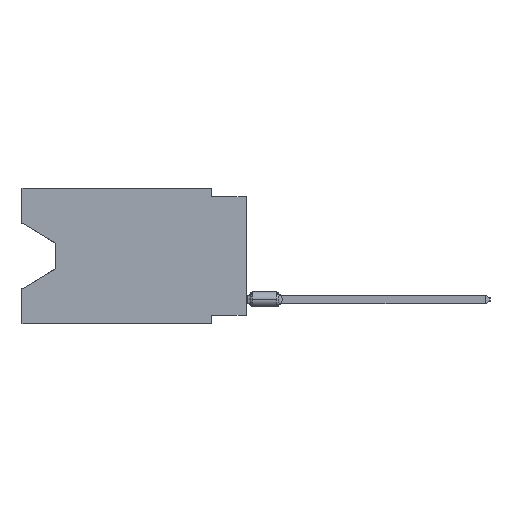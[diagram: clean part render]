
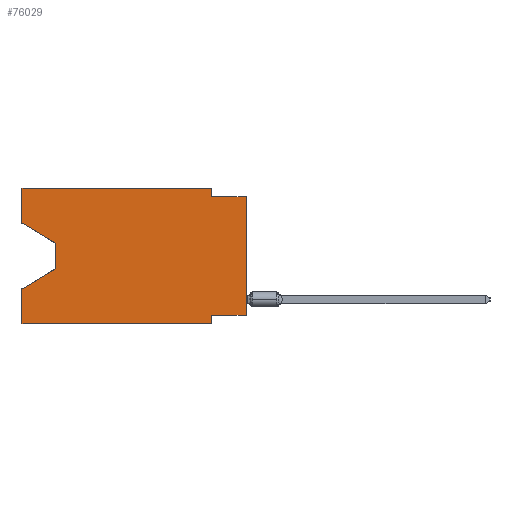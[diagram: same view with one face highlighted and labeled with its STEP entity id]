
A CAD part, left-side view. The second image highlights one B-rep face of the part: STEP entity #76029.
In plain terms, the highlighted planar face has unit normal (-1, 0, 0).
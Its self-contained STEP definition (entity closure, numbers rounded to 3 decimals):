
#23 = EDGE_CURVE ( 'NONE', #37314, #13199, #79784, .T. ) ;
#1327 = VECTOR ( 'NONE', #41392, 1000. ) ;
#2530 = VERTEX_POINT ( 'NONE', #23302 ) ;
#3319 = VERTEX_POINT ( 'NONE', #65923 ) ;
#4534 = VERTEX_POINT ( 'NONE', #23114 ) ;
#5900 = VECTOR ( 'NONE', #79385, 1000. ) ;
#6342 = LINE ( 'NONE', #75004, #16900 ) ;
#7025 = LINE ( 'NONE', #39284, #61425 ) ;
#7701 = EDGE_CURVE ( 'NONE', #2530, #56738, #6342, .T. ) ;
#9092 = LINE ( 'NONE', #40565, #30759 ) ;
#10693 = LINE ( 'NONE', #35314, #20684 ) ;
#11210 = CARTESIAN_POINT ( 'NONE',  ( 0., 16.383, 0. ) ) ;
#12800 = DIRECTION ( 'NONE',  ( 0., 0., 1. ) ) ;
#13199 = VERTEX_POINT ( 'NONE', #54015 ) ;
#13391 = VERTEX_POINT ( 'NONE', #25727 ) ;
#14161 = DIRECTION ( 'NONE',  ( 0., 0., -1. ) ) ;
#15362 = CARTESIAN_POINT ( 'NONE',  ( 0., 0., -0.635 ) ) ;
#16900 = VECTOR ( 'NONE', #24921, 1000. ) ;
#17189 = LINE ( 'NONE', #23638, #78007 ) ;
#18224 = PLANE ( 'NONE',  #79204 ) ;
#18334 = EDGE_CURVE ( 'NONE', #4534, #2530, #60759, .T. ) ;
#20684 = VECTOR ( 'NONE', #71680, 1000. ) ;
#20814 = DIRECTION ( 'NONE',  ( 0., 0.855, -0.519 ) ) ;
#21112 = VERTEX_POINT ( 'NONE', #76493 ) ;
#21815 = VERTEX_POINT ( 'NONE', #11210 ) ;
#22926 = ORIENTED_EDGE ( 'NONE', *, *, #48406, .T. ) ;
#23114 = CARTESIAN_POINT ( 'NONE',  ( 0., 0., -9.271 ) ) ;
#23302 = CARTESIAN_POINT ( 'NONE',  ( 0., 2.54, -9.271 ) ) ;
#23452 = EDGE_CURVE ( 'NONE', #35636, #56738, #17189, .T. ) ;
#23604 = CARTESIAN_POINT ( 'NONE',  ( 0., 16.383, 0. ) ) ;
#23638 = CARTESIAN_POINT ( 'NONE',  ( 0., 16.383, -9.906 ) ) ;
#24279 = CARTESIAN_POINT ( 'NONE',  ( 0., 16.383, -2.546 ) ) ;
#24784 = EDGE_CURVE ( 'NONE', #21815, #21112, #53457, .T. ) ;
#24921 = DIRECTION ( 'NONE',  ( 0., 0., -1. ) ) ;
#25691 = VECTOR ( 'NONE', #42170, 1000. ) ;
#25727 = CARTESIAN_POINT ( 'NONE',  ( 0., 2.54, -0.635 ) ) ;
#27282 = VECTOR ( 'NONE', #12800, 1000. ) ;
#28426 = CARTESIAN_POINT ( 'NONE',  ( 0., 16.383, 0. ) ) ;
#28450 = CARTESIAN_POINT ( 'NONE',  ( 0., 16.383, -9.906 ) ) ;
#29089 = EDGE_CURVE ( 'NONE', #21112, #13391, #39169, .T. ) ;
#30505 = DIRECTION ( 'NONE',  ( 0., -1., 0. ) ) ;
#30759 = VECTOR ( 'NONE', #20814, 1000. ) ;
#32301 = ORIENTED_EDGE ( 'NONE', *, *, #23452, .T. ) ;
#33274 = ORIENTED_EDGE ( 'NONE', *, *, #40555, .T. ) ;
#35314 = CARTESIAN_POINT ( 'NONE',  ( 0., 0., 0. ) ) ;
#35636 = VERTEX_POINT ( 'NONE', #28450 ) ;
#37314 = VERTEX_POINT ( 'NONE', #24279 ) ;
#37596 = DIRECTION ( 'NONE',  ( 1., 0., 0. ) ) ;
#39169 = LINE ( 'NONE', #45250, #62645 ) ;
#39284 = CARTESIAN_POINT ( 'NONE',  ( 0., 0., -0.635 ) ) ;
#39684 = ORIENTED_EDGE ( 'NONE', *, *, #18334, .F. ) ;
#40555 = EDGE_CURVE ( 'NONE', #3319, #69818, #9092, .T. ) ;
#40565 = CARTESIAN_POINT ( 'NONE',  ( 0., 13.97, -5.893 ) ) ;
#40620 = EDGE_LOOP ( 'NONE', ( #45428, #63858, #33274, #63310, #32301, #43025, #39684, #22926, #68552, #58612, #60111, #71440 ) ) ;
#41392 = DIRECTION ( 'NONE',  ( 0., 0., 1. ) ) ;
#42170 = DIRECTION ( 'NONE',  ( 0., 1., 0. ) ) ;
#42705 = CARTESIAN_POINT ( 'NONE',  ( 0., 16.383, 0. ) ) ;
#43025 = ORIENTED_EDGE ( 'NONE', *, *, #7701, .F. ) ;
#43659 = FACE_OUTER_BOUND ( 'NONE', #40620, .T. ) ;
#45250 = CARTESIAN_POINT ( 'NONE',  ( 0., 2.54, 0. ) ) ;
#45428 = ORIENTED_EDGE ( 'NONE', *, *, #23, .T. ) ;
#47391 = DIRECTION ( 'NONE',  ( 0., -1., 0. ) ) ;
#48353 = LINE ( 'NONE', #42705, #27282 ) ;
#48368 = EDGE_CURVE ( 'NONE', #35636, #69818, #78149, .T. ) ;
#48406 = EDGE_CURVE ( 'NONE', #4534, #64864, #10693, .T. ) ;
#51576 = LINE ( 'NONE', #63318, #63236 ) ;
#53457 = LINE ( 'NONE', #28426, #67868 ) ;
#54015 = CARTESIAN_POINT ( 'NONE',  ( 0., 13.97, -4.013 ) ) ;
#55732 = EDGE_CURVE ( 'NONE', #13199, #3319, #51576, .T. ) ;
#56738 = VERTEX_POINT ( 'NONE', #60948 ) ;
#58612 = ORIENTED_EDGE ( 'NONE', *, *, #29089, .F. ) ;
#59843 = CARTESIAN_POINT ( 'NONE',  ( 0., 16.383, -7.36 ) ) ;
#59945 = CARTESIAN_POINT ( 'NONE',  ( 0., 0., -9.271 ) ) ;
#60111 = ORIENTED_EDGE ( 'NONE', *, *, #24784, .F. ) ;
#60759 = LINE ( 'NONE', #59945, #25691 ) ;
#60948 = CARTESIAN_POINT ( 'NONE',  ( 0., 2.54, -9.906 ) ) ;
#61425 = VECTOR ( 'NONE', #63932, 1000. ) ;
#62244 = DIRECTION ( 'NONE',  ( 0., 0., -1. ) ) ;
#62645 = VECTOR ( 'NONE', #14161, 1000. ) ;
#63236 = VECTOR ( 'NONE', #76241, 1000. ) ;
#63310 = ORIENTED_EDGE ( 'NONE', *, *, #48368, .F. ) ;
#63318 = CARTESIAN_POINT ( 'NONE',  ( 0., 13.97, -4.013 ) ) ;
#63858 = ORIENTED_EDGE ( 'NONE', *, *, #55732, .T. ) ;
#63932 = DIRECTION ( 'NONE',  ( 0., -1., 0. ) ) ;
#64864 = VERTEX_POINT ( 'NONE', #15362 ) ;
#65498 = EDGE_CURVE ( 'NONE', #37314, #21815, #48353, .T. ) ;
#65923 = CARTESIAN_POINT ( 'NONE',  ( 0., 13.97, -5.893 ) ) ;
#67868 = VECTOR ( 'NONE', #47391, 1000. ) ;
#68035 = CARTESIAN_POINT ( 'NONE',  ( 0., 16.383, -2.546 ) ) ;
#68289 = CARTESIAN_POINT ( 'NONE',  ( 0., 16.383, 0. ) ) ;
#68552 = ORIENTED_EDGE ( 'NONE', *, *, #78568, .F. ) ;
#69818 = VERTEX_POINT ( 'NONE', #59843 ) ;
#71440 = ORIENTED_EDGE ( 'NONE', *, *, #65498, .F. ) ;
#71680 = DIRECTION ( 'NONE',  ( 0., 0., 1. ) ) ;
#75004 = CARTESIAN_POINT ( 'NONE',  ( 0., 2.54, -9.906 ) ) ;
#76029 = ADVANCED_FACE ( 'NONE', ( #43659 ), #18224, .F. ) ;
#76241 = DIRECTION ( 'NONE',  ( 0., 0., -1. ) ) ;
#76493 = CARTESIAN_POINT ( 'NONE',  ( 0., 2.54, 0. ) ) ;
#78007 = VECTOR ( 'NONE', #30505, 1000. ) ;
#78149 = LINE ( 'NONE', #23604, #1327 ) ;
#78568 = EDGE_CURVE ( 'NONE', #13391, #64864, #7025, .T. ) ;
#79204 = AXIS2_PLACEMENT_3D ( 'NONE', #68289, #37596, #62244 ) ;
#79385 = DIRECTION ( 'NONE',  ( 0., -0.855, -0.519 ) ) ;
#79784 = LINE ( 'NONE', #68035, #5900 ) ;
